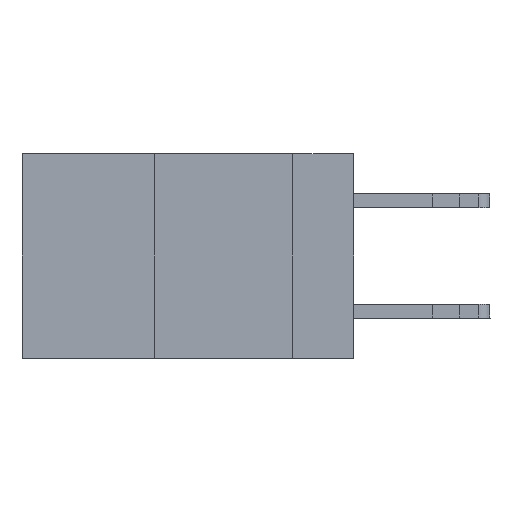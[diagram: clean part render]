
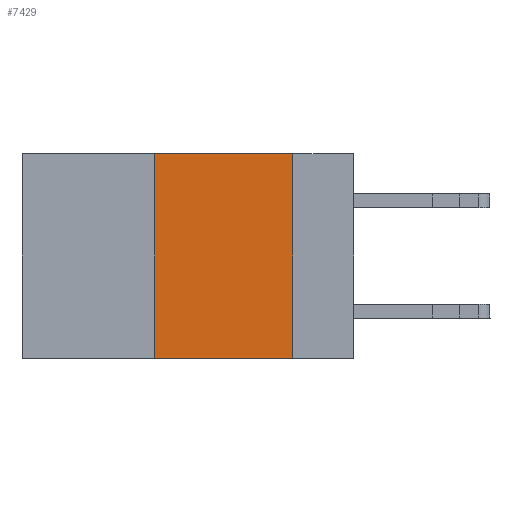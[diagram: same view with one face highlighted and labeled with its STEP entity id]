
A CAD part, left-side view. The second image highlights one B-rep face of the part: STEP entity #7429.
In plain terms, the highlighted planar face has unit normal (-1, 0, 0).
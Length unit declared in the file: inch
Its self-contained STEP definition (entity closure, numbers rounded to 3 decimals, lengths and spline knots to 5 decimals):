
#160 = VECTOR ( 'NONE', #337, 39.37008 ) ;
#292 = EDGE_CURVE ( 'NONE', #10520, #2665, #20662, .T. ) ;
#337 = DIRECTION ( 'NONE',  ( 0., 0., -1. ) ) ;
#645 = ORIENTED_EDGE ( 'NONE', *, *, #21791, .F. ) ;
#790 = ORIENTED_EDGE ( 'NONE', *, *, #6790, .T. ) ;
#1477 = DIRECTION ( 'NONE',  ( 0., -1., 0. ) ) ;
#2249 = CARTESIAN_POINT ( 'NONE',  ( 0., 0.6, 0. ) ) ;
#2665 = VERTEX_POINT ( 'NONE', #8806 ) ;
#3135 = EDGE_LOOP ( 'NONE', ( #19513, #20601, #645, #790 ) ) ;
#3505 = AXIS2_PLACEMENT_3D ( 'NONE', #7294, #21084, #10827 ) ;
#4362 = LINE ( 'NONE', #21195, #160 ) ;
#4801 = VERTEX_POINT ( 'NONE', #7396 ) ;
#6790 = EDGE_CURVE ( 'NONE', #4801, #12884, #17883, .T. ) ;
#7294 = CARTESIAN_POINT ( 'NONE',  ( 0., 0.6, 0. ) ) ;
#7396 = CARTESIAN_POINT ( 'NONE',  ( 0., 0.36, -0.37 ) ) ;
#7429 = ADVANCED_FACE ( 'NONE', ( #18125 ), #14172, .F. ) ;
#8772 = VECTOR ( 'NONE', #14050, 39.37008 ) ;
#8806 = CARTESIAN_POINT ( 'NONE',  ( 0., 0.11, 0. ) ) ;
#10520 = VERTEX_POINT ( 'NONE', #15857 ) ;
#10827 = DIRECTION ( 'NONE',  ( 0., 0., -1. ) ) ;
#11006 = VECTOR ( 'NONE', #1477, 39.37008 ) ;
#11702 = DIRECTION ( 'NONE',  ( 0., 0., 1. ) ) ;
#12884 = VERTEX_POINT ( 'NONE', #15729 ) ;
#14050 = DIRECTION ( 'NONE',  ( 0., -1., 0. ) ) ;
#14172 = PLANE ( 'NONE',  #3505 ) ;
#15056 = CARTESIAN_POINT ( 'NONE',  ( 0., 0.36, 0. ) ) ;
#15729 = CARTESIAN_POINT ( 'NONE',  ( 0., 0.11, -0.37 ) ) ;
#15857 = CARTESIAN_POINT ( 'NONE',  ( 0., 0.36, 0. ) ) ;
#17883 = LINE ( 'NONE', #20970, #8772 ) ;
#18125 = FACE_OUTER_BOUND ( 'NONE', #3135, .T. ) ;
#19513 = ORIENTED_EDGE ( 'NONE', *, *, #22118, .F. ) ;
#20601 = ORIENTED_EDGE ( 'NONE', *, *, #292, .F. ) ;
#20662 = LINE ( 'NONE', #2249, #11006 ) ;
#20970 = CARTESIAN_POINT ( 'NONE',  ( 0., 0.6, -0.37 ) ) ;
#21084 = DIRECTION ( 'NONE',  ( 1., 0., 0. ) ) ;
#21168 = LINE ( 'NONE', #15056, #21675 ) ;
#21195 = CARTESIAN_POINT ( 'NONE',  ( 0., 0.11, 0. ) ) ;
#21675 = VECTOR ( 'NONE', #11702, 39.37008 ) ;
#21791 = EDGE_CURVE ( 'NONE', #4801, #10520, #21168, .T. ) ;
#22118 = EDGE_CURVE ( 'NONE', #2665, #12884, #4362, .T. ) ;
